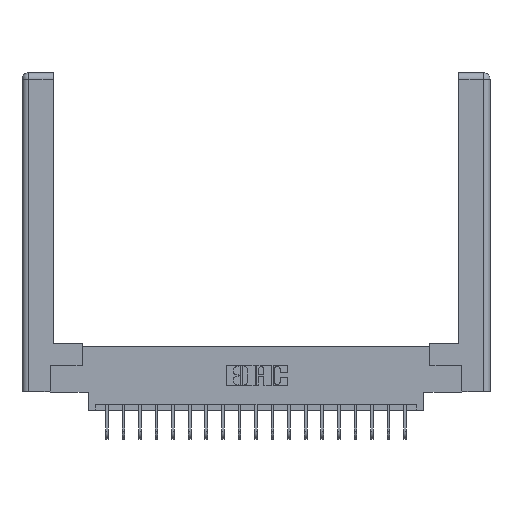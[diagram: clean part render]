
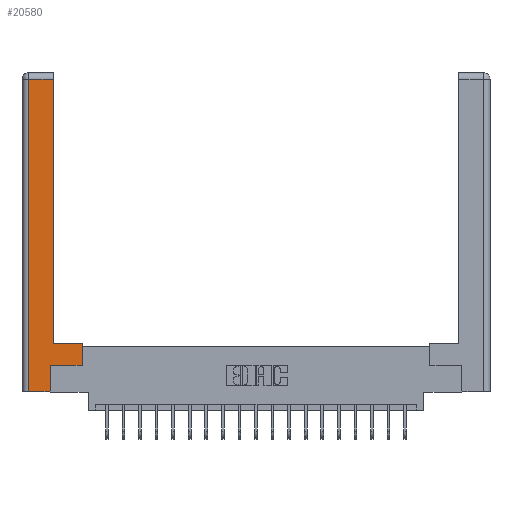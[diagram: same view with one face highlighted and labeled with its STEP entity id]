
A CAD part, top view. The second image highlights one B-rep face of the part: STEP entity #20580.
In plain terms, the highlighted planar face has unit normal (0, 0, 1).
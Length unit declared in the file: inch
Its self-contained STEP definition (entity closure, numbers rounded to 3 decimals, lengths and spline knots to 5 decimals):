
#1024 = VERTEX_POINT ( 'NONE', #5957 ) ;
#1805 = ORIENTED_EDGE ( 'NONE', *, *, #17166, .T. ) ;
#1957 = ORIENTED_EDGE ( 'NONE', *, *, #21618, .T. ) ;
#1997 = LINE ( 'NONE', #13945, #5211 ) ;
#2422 = CARTESIAN_POINT ( 'NONE',  ( 0.295, 3., 0. ) ) ;
#2586 = DIRECTION ( 'NONE',  ( 0., 0., -1. ) ) ;
#2997 = VERTEX_POINT ( 'NONE', #11676 ) ;
#3444 = DIRECTION ( 'NONE',  ( -1., 0., 0. ) ) ;
#3603 = VERTEX_POINT ( 'NONE', #12182 ) ;
#3774 = DIRECTION ( 'NONE',  ( 1., 0., 0. ) ) ;
#3823 = EDGE_CURVE ( 'NONE', #2997, #3996, #7830, .T. ) ;
#3882 = VECTOR ( 'NONE', #4155, 39.37008 ) ;
#3996 = VERTEX_POINT ( 'NONE', #19956 ) ;
#4155 = DIRECTION ( 'NONE',  ( 0., 1., 0. ) ) ;
#5211 = VECTOR ( 'NONE', #19113, 39.37008 ) ;
#5459 = EDGE_CURVE ( 'NONE', #3996, #15172, #12338, .T. ) ;
#5946 = LINE ( 'NONE', #10725, #21047 ) ;
#5957 = CARTESIAN_POINT ( 'NONE',  ( 0.295, 0.45, 0. ) ) ;
#6124 = PLANE ( 'NONE',  #20880 ) ;
#6145 = EDGE_CURVE ( 'NONE', #15241, #1024, #21337, .T. ) ;
#6816 = EDGE_CURVE ( 'NONE', #15172, #11393, #5946, .T. ) ;
#7113 = CARTESIAN_POINT ( 'NONE',  ( 0.0615, 2.94, 0. ) ) ;
#7157 = VECTOR ( 'NONE', #17641, 39.37008 ) ;
#7321 = CARTESIAN_POINT ( 'NONE',  ( 0.565, 0.45, 0. ) ) ;
#7676 = LINE ( 'NONE', #9191, #7157 ) ;
#7830 = LINE ( 'NONE', #17949, #9699 ) ;
#7842 = DIRECTION ( 'NONE',  ( 0., 1., 0. ) ) ;
#8130 = ORIENTED_EDGE ( 'NONE', *, *, #6816, .T. ) ;
#8688 = ORIENTED_EDGE ( 'NONE', *, *, #6145, .T. ) ;
#9050 = ORIENTED_EDGE ( 'NONE', *, *, #5459, .T. ) ;
#9191 = CARTESIAN_POINT ( 'NONE',  ( 0.565, 0.45, 0. ) ) ;
#9564 = ORIENTED_EDGE ( 'NONE', *, *, #3823, .T. ) ;
#9588 = DIRECTION ( 'NONE',  ( -1., 0., 0. ) ) ;
#9699 = VECTOR ( 'NONE', #17883, 39.37008 ) ;
#10725 = CARTESIAN_POINT ( 'NONE',  ( 0.565, 0.245, 0. ) ) ;
#11099 = VECTOR ( 'NONE', #3444, 39.37008 ) ;
#11393 = VERTEX_POINT ( 'NONE', #15200 ) ;
#11676 = CARTESIAN_POINT ( 'NONE',  ( 0.0615, 0., 0. ) ) ;
#12019 = VERTEX_POINT ( 'NONE', #13512 ) ;
#12153 = EDGE_LOOP ( 'NONE', ( #15922, #15999, #1957, #9564, #9050, #8130, #1805, #8688 ) ) ;
#12182 = CARTESIAN_POINT ( 'NONE',  ( 0.295, 2.94, 0. ) ) ;
#12338 = LINE ( 'NONE', #19647, #16926 ) ;
#13512 = CARTESIAN_POINT ( 'NONE',  ( 0.0615, 2.94, 0. ) ) ;
#13945 = CARTESIAN_POINT ( 'NONE',  ( 0.0615, 0., 0. ) ) ;
#13958 = VECTOR ( 'NONE', #19127, 39.37008 ) ;
#15172 = VERTEX_POINT ( 'NONE', #17264 ) ;
#15200 = CARTESIAN_POINT ( 'NONE',  ( 0.565, 0.245, 0. ) ) ;
#15241 = VERTEX_POINT ( 'NONE', #7321 ) ;
#15288 = EDGE_CURVE ( 'NONE', #3603, #12019, #21742, .T. ) ;
#15922 = ORIENTED_EDGE ( 'NONE', *, *, #21193, .T. ) ;
#15999 = ORIENTED_EDGE ( 'NONE', *, *, #15288, .T. ) ;
#16558 = CARTESIAN_POINT ( 'NONE',  ( 0.295, 0.45, 0. ) ) ;
#16926 = VECTOR ( 'NONE', #7842, 39.37008 ) ;
#17166 = EDGE_CURVE ( 'NONE', #11393, #15241, #7676, .T. ) ;
#17264 = CARTESIAN_POINT ( 'NONE',  ( 0.265, 0.245, 0. ) ) ;
#17641 = DIRECTION ( 'NONE',  ( 0., 1., 0. ) ) ;
#17883 = DIRECTION ( 'NONE',  ( 1., 0., 0. ) ) ;
#17949 = CARTESIAN_POINT ( 'NONE',  ( 0.265, 0., 0. ) ) ;
#18413 = LINE ( 'NONE', #2422, #3882 ) ;
#18458 = FACE_OUTER_BOUND ( 'NONE', #12153, .T. ) ;
#19113 = DIRECTION ( 'NONE',  ( 0., -1., 0. ) ) ;
#19127 = DIRECTION ( 'NONE',  ( -1., 0., 0. ) ) ;
#19647 = CARTESIAN_POINT ( 'NONE',  ( 0.265, 0.245, 0. ) ) ;
#19810 = CARTESIAN_POINT ( 'NONE',  ( 0., 0., 0. ) ) ;
#19956 = CARTESIAN_POINT ( 'NONE',  ( 0.265, 0., 0. ) ) ;
#20580 = ADVANCED_FACE ( 'NONE', ( #18458 ), #6124, .F. ) ;
#20880 = AXIS2_PLACEMENT_3D ( 'NONE', #19810, #2586, #9588 ) ;
#21047 = VECTOR ( 'NONE', #3774, 39.37008 ) ;
#21193 = EDGE_CURVE ( 'NONE', #1024, #3603, #18413, .T. ) ;
#21337 = LINE ( 'NONE', #16558, #11099 ) ;
#21618 = EDGE_CURVE ( 'NONE', #12019, #2997, #1997, .T. ) ;
#21742 = LINE ( 'NONE', #7113, #13958 ) ;
